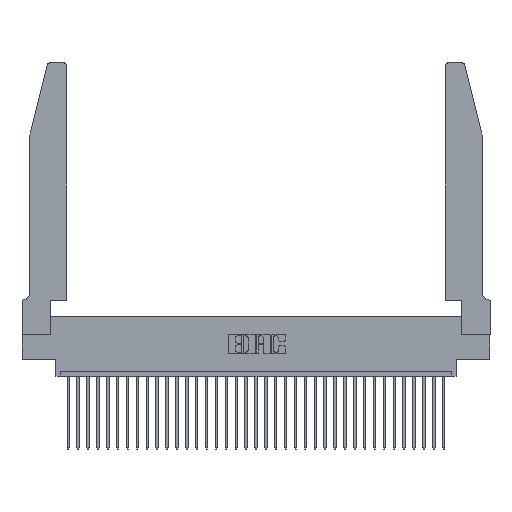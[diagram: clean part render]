
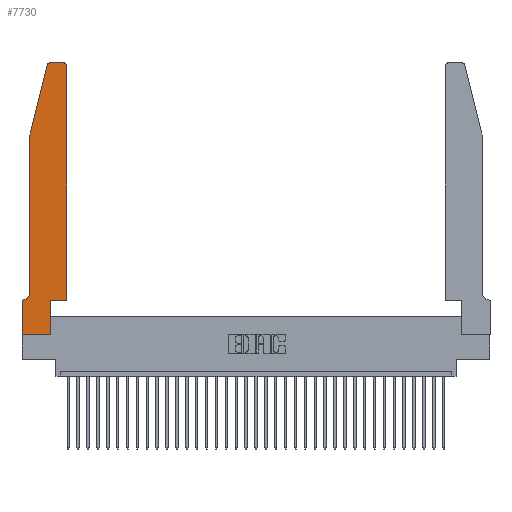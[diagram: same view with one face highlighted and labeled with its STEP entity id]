
A CAD part, top view. The second image highlights one B-rep face of the part: STEP entity #7730.
In plain terms, the highlighted planar face has unit normal (0, 0, 1).
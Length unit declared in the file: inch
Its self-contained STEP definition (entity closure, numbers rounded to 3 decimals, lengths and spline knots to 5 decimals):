
#291 = CARTESIAN_POINT ( 'NONE',  ( 0.4205, 2.75, 0.37 ) ) ;
#1395 = VECTOR ( 'NONE', #27828, 39.37008 ) ;
#1472 = ORIENTED_EDGE ( 'NONE', *, *, #24804, .T. ) ;
#1527 = CARTESIAN_POINT ( 'NONE',  ( 0.2865, 0., 0.37 ) ) ;
#2568 = DIRECTION ( 'NONE',  ( 1., 0., 0. ) ) ;
#2753 = VERTEX_POINT ( 'NONE', #1527 ) ;
#3541 = EDGE_CURVE ( 'NONE', #33777, #30726, #26202, .T. ) ;
#3826 = VERTEX_POINT ( 'NONE', #9026 ) ;
#3940 = LINE ( 'NONE', #13797, #19350 ) ;
#4718 = LINE ( 'NONE', #9795, #15210 ) ;
#4787 = CARTESIAN_POINT ( 'NONE',  ( 0., 0.35, 0.37 ) ) ;
#5210 = ORIENTED_EDGE ( 'NONE', *, *, #11190, .T. ) ;
#5481 = EDGE_CURVE ( 'NONE', #10855, #3826, #10495, .T. ) ;
#6280 = DIRECTION ( 'NONE',  ( 0., 1., 0. ) ) ;
#6518 = DIRECTION ( 'NONE',  ( 0., 0., -1. ) ) ;
#6636 = FACE_OUTER_BOUND ( 'NONE', #32780, .T. ) ;
#6712 = DIRECTION ( 'NONE',  ( 0., -1., 0. ) ) ;
#7454 = CARTESIAN_POINT ( 'NONE',  ( 0.4505, 0.35, 0.37 ) ) ;
#7671 = VECTOR ( 'NONE', #18010, 39.37008 ) ;
#7730 = ADVANCED_FACE ( 'NONE', ( #6636 ), #31814, .T. ) ;
#8979 = ORIENTED_EDGE ( 'NONE', *, *, #5481, .T. ) ;
#9026 = CARTESIAN_POINT ( 'NONE',  ( 0., 0.35, 0.37 ) ) ;
#9125 = CARTESIAN_POINT ( 'NONE',  ( 0.0755, 2., 0.37 ) ) ;
#9184 = DIRECTION ( 'NONE',  ( -1., 0., 0. ) ) ;
#9244 = VECTOR ( 'NONE', #24761, 39.37008 ) ;
#9795 = CARTESIAN_POINT ( 'NONE',  ( 0., 0., 0.37 ) ) ;
#10017 = EDGE_CURVE ( 'NONE', #14903, #31937, #3940, .T. ) ;
#10093 = DIRECTION ( 'NONE',  ( 1., 0., 0. ) ) ;
#10226 = EDGE_CURVE ( 'NONE', #27031, #20152, #31587, .T. ) ;
#10350 = DIRECTION ( 'NONE',  ( 0., 0., 1. ) ) ;
#10382 = EDGE_CURVE ( 'NONE', #2753, #33777, #25236, .T. ) ;
#10438 = EDGE_CURVE ( 'NONE', #23175, #27031, #18531, .T. ) ;
#10495 = LINE ( 'NONE', #21378, #9244 ) ;
#10543 = DIRECTION ( 'NONE',  ( 1., 0., 0. ) ) ;
#10787 = ORIENTED_EDGE ( 'NONE', *, *, #25184, .T. ) ;
#10855 = VERTEX_POINT ( 'NONE', #25122 ) ;
#10865 = CARTESIAN_POINT ( 'NONE',  ( 0.0755, 0.42, 0.37 ) ) ;
#10884 = ORIENTED_EDGE ( 'NONE', *, *, #10017, .T. ) ;
#11190 = EDGE_CURVE ( 'NONE', #24693, #2753, #12189, .T. ) ;
#11463 = ORIENTED_EDGE ( 'NONE', *, *, #25911, .T. ) ;
#12189 = LINE ( 'NONE', #26412, #25631 ) ;
#12893 = CARTESIAN_POINT ( 'NONE',  ( 0.284, 2.75, 0.37 ) ) ;
#13791 = CARTESIAN_POINT ( 'NONE',  ( 0.4505, 2.72, 0.37 ) ) ;
#13797 = CARTESIAN_POINT ( 'NONE',  ( 0.0755, 2., 0.37 ) ) ;
#13964 = CARTESIAN_POINT ( 'NONE',  ( 0.0755, 2., 0.37 ) ) ;
#14170 = AXIS2_PLACEMENT_3D ( 'NONE', #4787, #10350, #23505 ) ;
#14500 = ORIENTED_EDGE ( 'NONE', *, *, #10438, .T. ) ;
#14678 = VECTOR ( 'NONE', #6712, 39.37008 ) ;
#14739 = CARTESIAN_POINT ( 'NONE',  ( 0.2605, 2.75, 0.37 ) ) ;
#14764 = CARTESIAN_POINT ( 'NONE',  ( 0.4205, 2.72, 0.37 ) ) ;
#14903 = VERTEX_POINT ( 'NONE', #17534 ) ;
#15007 = DIRECTION ( 'NONE',  ( 1., 0., 0. ) ) ;
#15210 = VECTOR ( 'NONE', #31515, 39.37008 ) ;
#15268 = CARTESIAN_POINT ( 'NONE',  ( 0.2865, 0.35, 0.37 ) ) ;
#15536 = LINE ( 'NONE', #9125, #14678 ) ;
#16029 = AXIS2_PLACEMENT_3D ( 'NONE', #16425, #26187, #10093 ) ;
#16425 = CARTESIAN_POINT ( 'NONE',  ( 0.284, 2.72, 0.37 ) ) ;
#16675 = CARTESIAN_POINT ( 'NONE',  ( 0.2865, 0.35, 0.37 ) ) ;
#17456 = DIRECTION ( 'NONE',  ( 0., 0., 1. ) ) ;
#17534 = CARTESIAN_POINT ( 'NONE',  ( 0.25487, 2.72718, 0.37 ) ) ;
#18010 = DIRECTION ( 'NONE',  ( 0., 1., 0. ) ) ;
#18052 = VECTOR ( 'NONE', #6280, 39.37008 ) ;
#18531 = CIRCLE ( 'NONE', #24333, 0.03 ) ;
#18880 = CIRCLE ( 'NONE', #16029, 0.03 ) ;
#19350 = VECTOR ( 'NONE', #21867, 39.37008 ) ;
#19536 = EDGE_CURVE ( 'NONE', #31937, #27682, #15536, .T. ) ;
#20152 = VERTEX_POINT ( 'NONE', #12893 ) ;
#21378 = CARTESIAN_POINT ( 'NONE',  ( 0.0755, 0.35, 0.37 ) ) ;
#21867 = DIRECTION ( 'NONE',  ( -0.239, -0.971, 0. ) ) ;
#22146 = ORIENTED_EDGE ( 'NONE', *, *, #19536, .T. ) ;
#22198 = CARTESIAN_POINT ( 'NONE',  ( 0.4505, 0.35, 0.37 ) ) ;
#23175 = VERTEX_POINT ( 'NONE', #13791 ) ;
#23505 = DIRECTION ( 'NONE',  ( 1., 0., 0. ) ) ;
#23648 = ORIENTED_EDGE ( 'NONE', *, *, #10382, .T. ) ;
#24333 = AXIS2_PLACEMENT_3D ( 'NONE', #14764, #17456, #15007 ) ;
#24693 = VERTEX_POINT ( 'NONE', #29080 ) ;
#24761 = DIRECTION ( 'NONE',  ( -1., 0., 0. ) ) ;
#24804 = EDGE_CURVE ( 'NONE', #3826, #24693, #4718, .T. ) ;
#25122 = CARTESIAN_POINT ( 'NONE',  ( 0.0055, 0.35, 0.37 ) ) ;
#25162 = ORIENTED_EDGE ( 'NONE', *, *, #33261, .T. ) ;
#25184 = EDGE_CURVE ( 'NONE', #20152, #14903, #18880, .T. ) ;
#25236 = LINE ( 'NONE', #15268, #7671 ) ;
#25631 = VECTOR ( 'NONE', #10543, 39.37008 ) ;
#25868 = CIRCLE ( 'NONE', #29006, 0.07 ) ;
#25911 = EDGE_CURVE ( 'NONE', #30726, #23175, #28073, .T. ) ;
#26187 = DIRECTION ( 'NONE',  ( 0., 0., 1. ) ) ;
#26202 = LINE ( 'NONE', #26769, #32872 ) ;
#26412 = CARTESIAN_POINT ( 'NONE',  ( 0., 0., 0.37 ) ) ;
#26769 = CARTESIAN_POINT ( 'NONE',  ( 0.4505, 0.35, 0.37 ) ) ;
#27031 = VERTEX_POINT ( 'NONE', #291 ) ;
#27682 = VERTEX_POINT ( 'NONE', #10865 ) ;
#27828 = DIRECTION ( 'NONE',  ( -1., 0., 0. ) ) ;
#27947 = ORIENTED_EDGE ( 'NONE', *, *, #3541, .T. ) ;
#28073 = LINE ( 'NONE', #22198, #18052 ) ;
#29006 = AXIS2_PLACEMENT_3D ( 'NONE', #33438, #6518, #9184 ) ;
#29080 = CARTESIAN_POINT ( 'NONE',  ( 0., 0., 0.37 ) ) ;
#30726 = VERTEX_POINT ( 'NONE', #7454 ) ;
#31515 = DIRECTION ( 'NONE',  ( 0., -1., 0. ) ) ;
#31587 = LINE ( 'NONE', #14739, #1395 ) ;
#31814 = PLANE ( 'NONE',  #14170 ) ;
#31937 = VERTEX_POINT ( 'NONE', #13964 ) ;
#32780 = EDGE_LOOP ( 'NONE', ( #33118, #10787, #10884, #22146, #25162, #8979, #1472, #5210, #23648, #27947, #11463, #14500 ) ) ;
#32872 = VECTOR ( 'NONE', #2568, 39.37008 ) ;
#33118 = ORIENTED_EDGE ( 'NONE', *, *, #10226, .T. ) ;
#33261 = EDGE_CURVE ( 'NONE', #27682, #10855, #25868, .T. ) ;
#33438 = CARTESIAN_POINT ( 'NONE',  ( 0.0055, 0.42, 0.37 ) ) ;
#33777 = VERTEX_POINT ( 'NONE', #16675 ) ;
